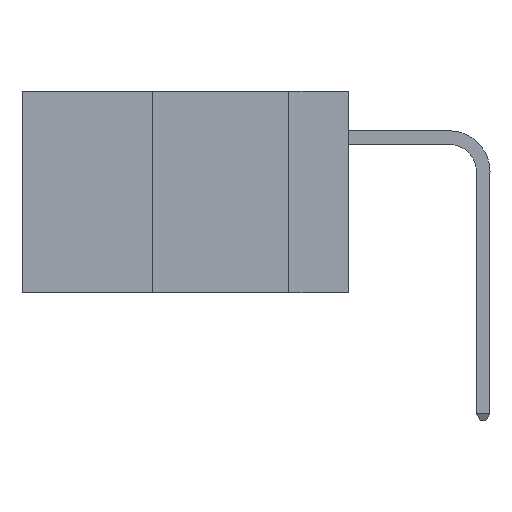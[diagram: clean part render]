
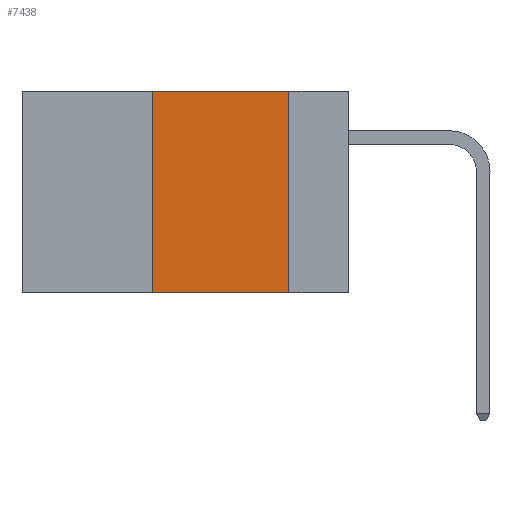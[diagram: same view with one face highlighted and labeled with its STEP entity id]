
A CAD part, left-side view. The second image highlights one B-rep face of the part: STEP entity #7438.
In plain terms, the highlighted planar face has unit normal (-1, 0, 0).
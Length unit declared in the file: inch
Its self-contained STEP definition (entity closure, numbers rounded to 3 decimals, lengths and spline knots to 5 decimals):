
#28 = ORIENTED_EDGE ( 'NONE', *, *, #17390, .F. ) ;
#152 = CARTESIAN_POINT ( 'NONE',  ( 0., 0.36, 0. ) ) ;
#519 = VERTEX_POINT ( 'NONE', #13241 ) ;
#630 = FACE_OUTER_BOUND ( 'NONE', #6695, .T. ) ;
#769 = DIRECTION ( 'NONE',  ( 0., 0., -1. ) ) ;
#773 = DIRECTION ( 'NONE',  ( 0., -1., 0. ) ) ;
#1257 = CARTESIAN_POINT ( 'NONE',  ( 0., 0.11, 0. ) ) ;
#1530 = AXIS2_PLACEMENT_3D ( 'NONE', #5446, #18277, #769 ) ;
#1844 = VERTEX_POINT ( 'NONE', #152 ) ;
#3824 = EDGE_CURVE ( 'NONE', #6685, #1844, #11453, .T. ) ;
#4784 = CARTESIAN_POINT ( 'NONE',  ( 0., 0.11, 0. ) ) ;
#5446 = CARTESIAN_POINT ( 'NONE',  ( 0., 0.6, 0. ) ) ;
#5507 = CARTESIAN_POINT ( 'NONE',  ( 0., 0.6, 0. ) ) ;
#6554 = CARTESIAN_POINT ( 'NONE',  ( 0., 0.36, -0.37 ) ) ;
#6685 = VERTEX_POINT ( 'NONE', #6554 ) ;
#6695 = EDGE_LOOP ( 'NONE', ( #15914, #28, #17153, #14539 ) ) ;
#6890 = LINE ( 'NONE', #4784, #14796 ) ;
#7438 = ADVANCED_FACE ( 'NONE', ( #630 ), #18075, .F. ) ;
#8111 = VECTOR ( 'NONE', #773, 39.37008 ) ;
#9402 = LINE ( 'NONE', #10260, #9897 ) ;
#9897 = VECTOR ( 'NONE', #13827, 39.37008 ) ;
#10082 = LINE ( 'NONE', #5507, #8111 ) ;
#10260 = CARTESIAN_POINT ( 'NONE',  ( 0., 0.6, -0.37 ) ) ;
#11453 = LINE ( 'NONE', #12555, #13721 ) ;
#12555 = CARTESIAN_POINT ( 'NONE',  ( 0., 0.36, 0. ) ) ;
#13241 = CARTESIAN_POINT ( 'NONE',  ( 0., 0.11, -0.37 ) ) ;
#13721 = VECTOR ( 'NONE', #20427, 39.37008 ) ;
#13827 = DIRECTION ( 'NONE',  ( 0., -1., 0. ) ) ;
#14045 = DIRECTION ( 'NONE',  ( 0., 0., -1. ) ) ;
#14539 = ORIENTED_EDGE ( 'NONE', *, *, #15993, .T. ) ;
#14796 = VECTOR ( 'NONE', #14045, 39.37008 ) ;
#15914 = ORIENTED_EDGE ( 'NONE', *, *, #18015, .F. ) ;
#15993 = EDGE_CURVE ( 'NONE', #6685, #519, #9402, .T. ) ;
#17153 = ORIENTED_EDGE ( 'NONE', *, *, #3824, .F. ) ;
#17390 = EDGE_CURVE ( 'NONE', #1844, #17776, #10082, .T. ) ;
#17776 = VERTEX_POINT ( 'NONE', #1257 ) ;
#18015 = EDGE_CURVE ( 'NONE', #17776, #519, #6890, .T. ) ;
#18075 = PLANE ( 'NONE',  #1530 ) ;
#18277 = DIRECTION ( 'NONE',  ( 1., 0., 0. ) ) ;
#20427 = DIRECTION ( 'NONE',  ( 0., 0., 1. ) ) ;
